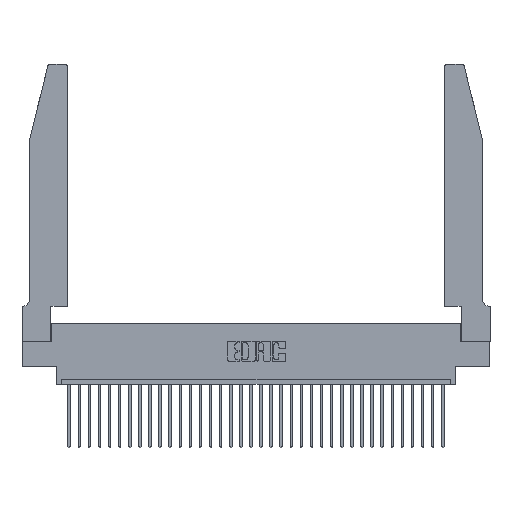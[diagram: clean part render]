
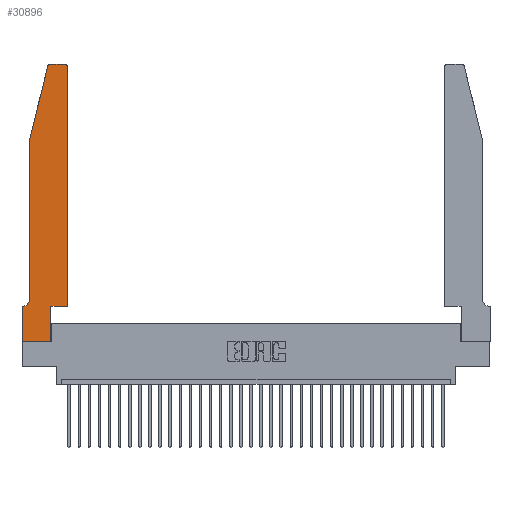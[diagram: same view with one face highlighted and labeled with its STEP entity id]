
A CAD part, top view. The second image highlights one B-rep face of the part: STEP entity #30896.
In plain terms, the highlighted planar face has unit normal (0, 0, 1).
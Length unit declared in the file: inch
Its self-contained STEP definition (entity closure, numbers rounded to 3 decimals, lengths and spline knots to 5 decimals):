
#323 = ORIENTED_EDGE ( 'NONE', *, *, #6262, .T. ) ;
#548 = CARTESIAN_POINT ( 'NONE',  ( 0., 0.35, 0.37 ) ) ;
#1758 = CARTESIAN_POINT ( 'NONE',  ( 0.2605, 2.75, 0.37 ) ) ;
#1901 = ORIENTED_EDGE ( 'NONE', *, *, #17291, .T. ) ;
#2048 = LINE ( 'NONE', #19809, #29930 ) ;
#3025 = CARTESIAN_POINT ( 'NONE',  ( 0.4505, 0.35, 0.37 ) ) ;
#3077 = VECTOR ( 'NONE', #15010, 39.37008 ) ;
#4801 = ORIENTED_EDGE ( 'NONE', *, *, #21239, .T. ) ;
#4842 = AXIS2_PLACEMENT_3D ( 'NONE', #17453, #14938, #9670 ) ;
#5233 = CARTESIAN_POINT ( 'NONE',  ( 0., 0., 0.37 ) ) ;
#5536 = CARTESIAN_POINT ( 'NONE',  ( 0.284, 2.75, 0.37 ) ) ;
#6262 = EDGE_CURVE ( 'NONE', #9962, #26421, #24761, .T. ) ;
#6484 = CARTESIAN_POINT ( 'NONE',  ( 0.2865, 0.35, 0.37 ) ) ;
#6710 = EDGE_CURVE ( 'NONE', #18694, #30263, #30972, .T. ) ;
#7005 = CARTESIAN_POINT ( 'NONE',  ( 0.0755, 2., 0.37 ) ) ;
#7041 = LINE ( 'NONE', #21211, #32491 ) ;
#7237 = LINE ( 'NONE', #7005, #3077 ) ;
#7329 = VERTEX_POINT ( 'NONE', #23504 ) ;
#7511 = VECTOR ( 'NONE', #21930, 39.37008 ) ;
#7669 = VERTEX_POINT ( 'NONE', #29012 ) ;
#8601 = CARTESIAN_POINT ( 'NONE',  ( 0.0055, 0.35, 0.37 ) ) ;
#8957 = CARTESIAN_POINT ( 'NONE',  ( 0., 0.35, 0.37 ) ) ;
#9670 = DIRECTION ( 'NONE',  ( 1., 0., 0. ) ) ;
#9942 = DIRECTION ( 'NONE',  ( 0., 0., -1. ) ) ;
#9962 = VERTEX_POINT ( 'NONE', #25231 ) ;
#11713 = EDGE_CURVE ( 'NONE', #13148, #16074, #14606, .T. ) ;
#12123 = EDGE_CURVE ( 'NONE', #7329, #9962, #7237, .T. ) ;
#12244 = CARTESIAN_POINT ( 'NONE',  ( 0.284, 2.72, 0.37 ) ) ;
#12958 = EDGE_CURVE ( 'NONE', #30263, #7669, #28097, .T. ) ;
#13148 = VERTEX_POINT ( 'NONE', #5233 ) ;
#14606 = LINE ( 'NONE', #18034, #32723 ) ;
#14609 = DIRECTION ( 'NONE',  ( -1., 0., 0. ) ) ;
#14776 = FACE_OUTER_BOUND ( 'NONE', #23522, .T. ) ;
#14906 = VERTEX_POINT ( 'NONE', #26393 ) ;
#14938 = DIRECTION ( 'NONE',  ( 0., 0., 1. ) ) ;
#15010 = DIRECTION ( 'NONE',  ( 0., -1., 0. ) ) ;
#15334 = CARTESIAN_POINT ( 'NONE',  ( 0.4505, 0.35, 0.37 ) ) ;
#15533 = AXIS2_PLACEMENT_3D ( 'NONE', #548, #31670, #31777 ) ;
#16074 = VERTEX_POINT ( 'NONE', #21889 ) ;
#16976 = VERTEX_POINT ( 'NONE', #18438 ) ;
#17291 = EDGE_CURVE ( 'NONE', #20902, #13148, #2048, .T. ) ;
#17453 = CARTESIAN_POINT ( 'NONE',  ( 0.4205, 2.72, 0.37 ) ) ;
#17735 = DIRECTION ( 'NONE',  ( 1., 0., 0. ) ) ;
#18034 = CARTESIAN_POINT ( 'NONE',  ( 0., 0., 0.37 ) ) ;
#18204 = ORIENTED_EDGE ( 'NONE', *, *, #19880, .T. ) ;
#18431 = ORIENTED_EDGE ( 'NONE', *, *, #30242, .T. ) ;
#18438 = CARTESIAN_POINT ( 'NONE',  ( 0.2865, 0.35, 0.37 ) ) ;
#18694 = VERTEX_POINT ( 'NONE', #30072 ) ;
#19527 = ORIENTED_EDGE ( 'NONE', *, *, #12123, .T. ) ;
#19809 = CARTESIAN_POINT ( 'NONE',  ( 0., 0., 0.37 ) ) ;
#19880 = EDGE_CURVE ( 'NONE', #7669, #7329, #26455, .T. ) ;
#20432 = LINE ( 'NONE', #15334, #30736 ) ;
#20662 = CARTESIAN_POINT ( 'NONE',  ( 0.4505, 0.35, 0.37 ) ) ;
#20738 = EDGE_CURVE ( 'NONE', #14906, #18694, #27635, .T. ) ;
#20902 = VERTEX_POINT ( 'NONE', #8957 ) ;
#21211 = CARTESIAN_POINT ( 'NONE',  ( 0.0755, 0.35, 0.37 ) ) ;
#21233 = ORIENTED_EDGE ( 'NONE', *, *, #6710, .T. ) ;
#21239 = EDGE_CURVE ( 'NONE', #16074, #16976, #27155, .T. ) ;
#21714 = ORIENTED_EDGE ( 'NONE', *, *, #12958, .T. ) ;
#21889 = CARTESIAN_POINT ( 'NONE',  ( 0.2865, 0., 0.37 ) ) ;
#21930 = DIRECTION ( 'NONE',  ( 0., 1., 0. ) ) ;
#21977 = ORIENTED_EDGE ( 'NONE', *, *, #32862, .T. ) ;
#22129 = LINE ( 'NONE', #3025, #27473 ) ;
#23030 = DIRECTION ( 'NONE',  ( 0., 1., 0. ) ) ;
#23504 = CARTESIAN_POINT ( 'NONE',  ( 0.0755, 2., 0.37 ) ) ;
#23522 = EDGE_LOOP ( 'NONE', ( #21233, #21714, #18204, #19527, #323, #18431, #1901, #33088, #4801, #23794, #21977, #28857 ) ) ;
#23794 = ORIENTED_EDGE ( 'NONE', *, *, #25539, .T. ) ;
#23922 = AXIS2_PLACEMENT_3D ( 'NONE', #28164, #9942, #14609 ) ;
#24001 = DIRECTION ( 'NONE',  ( 1., 0., 0. ) ) ;
#24679 = DIRECTION ( 'NONE',  ( -1., 0., 0. ) ) ;
#24761 = CIRCLE ( 'NONE', #23922, 0.07 ) ;
#24947 = DIRECTION ( 'NONE',  ( 0., -1., 0. ) ) ;
#25231 = CARTESIAN_POINT ( 'NONE',  ( 0.0755, 0.42, 0.37 ) ) ;
#25539 = EDGE_CURVE ( 'NONE', #16976, #32232, #22129, .T. ) ;
#26393 = CARTESIAN_POINT ( 'NONE',  ( 0.4505, 2.72, 0.37 ) ) ;
#26421 = VERTEX_POINT ( 'NONE', #8601 ) ;
#26455 = LINE ( 'NONE', #32218, #31445 ) ;
#27155 = LINE ( 'NONE', #6484, #7511 ) ;
#27473 = VECTOR ( 'NONE', #24001, 39.37008 ) ;
#27635 = CIRCLE ( 'NONE', #4842, 0.03 ) ;
#28097 = CIRCLE ( 'NONE', #32469, 0.03 ) ;
#28164 = CARTESIAN_POINT ( 'NONE',  ( 0.0055, 0.42, 0.37 ) ) ;
#28857 = ORIENTED_EDGE ( 'NONE', *, *, #20738, .T. ) ;
#29012 = CARTESIAN_POINT ( 'NONE',  ( 0.25487, 2.72718, 0.37 ) ) ;
#29198 = DIRECTION ( 'NONE',  ( -0.239, -0.971, 0. ) ) ;
#29573 = PLANE ( 'NONE',  #15533 ) ;
#29930 = VECTOR ( 'NONE', #24947, 39.37008 ) ;
#30072 = CARTESIAN_POINT ( 'NONE',  ( 0.4205, 2.75, 0.37 ) ) ;
#30242 = EDGE_CURVE ( 'NONE', #26421, #20902, #7041, .T. ) ;
#30263 = VERTEX_POINT ( 'NONE', #5536 ) ;
#30736 = VECTOR ( 'NONE', #23030, 39.37008 ) ;
#30896 = ADVANCED_FACE ( 'NONE', ( #14776 ), #29573, .T. ) ;
#30972 = LINE ( 'NONE', #1758, #32184 ) ;
#31445 = VECTOR ( 'NONE', #29198, 39.37008 ) ;
#31670 = DIRECTION ( 'NONE',  ( 0., 0., 1. ) ) ;
#31708 = DIRECTION ( 'NONE',  ( 1., 0., 0. ) ) ;
#31777 = DIRECTION ( 'NONE',  ( 1., 0., 0. ) ) ;
#32044 = DIRECTION ( 'NONE',  ( -1., 0., 0. ) ) ;
#32184 = VECTOR ( 'NONE', #24679, 39.37008 ) ;
#32218 = CARTESIAN_POINT ( 'NONE',  ( 0.0755, 2., 0.37 ) ) ;
#32232 = VERTEX_POINT ( 'NONE', #20662 ) ;
#32469 = AXIS2_PLACEMENT_3D ( 'NONE', #12244, #33273, #17735 ) ;
#32491 = VECTOR ( 'NONE', #32044, 39.37008 ) ;
#32723 = VECTOR ( 'NONE', #31708, 39.37008 ) ;
#32862 = EDGE_CURVE ( 'NONE', #32232, #14906, #20432, .T. ) ;
#33088 = ORIENTED_EDGE ( 'NONE', *, *, #11713, .T. ) ;
#33273 = DIRECTION ( 'NONE',  ( 0., 0., 1. ) ) ;
